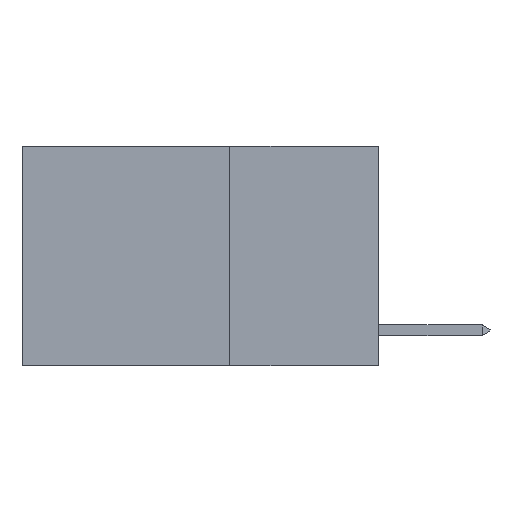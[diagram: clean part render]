
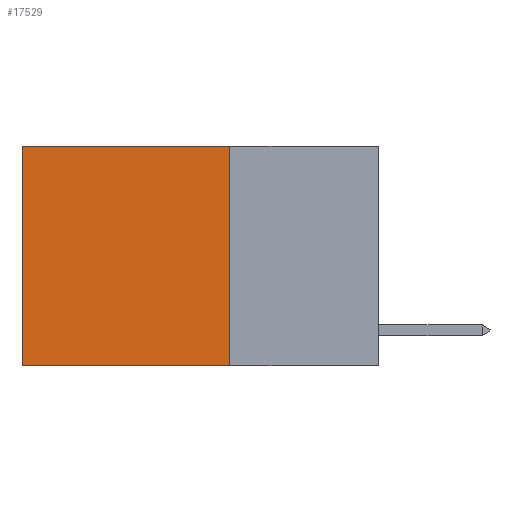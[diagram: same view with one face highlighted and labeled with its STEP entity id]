
A CAD part, left-side view. The second image highlights one B-rep face of the part: STEP entity #17529.
In plain terms, the highlighted planar face has unit normal (-1, 0, 0).
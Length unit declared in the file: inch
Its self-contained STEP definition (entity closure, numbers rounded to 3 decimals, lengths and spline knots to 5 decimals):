
#8 = CARTESIAN_POINT ( 'NONE',  ( 0.2625, 0.25, 0. ) ) ;
#123 = CARTESIAN_POINT ( 'NONE',  ( 0.2625, 0.6, 0. ) ) ;
#427 = VECTOR ( 'NONE', #13762, 39.37008 ) ;
#448 = DIRECTION ( 'NONE',  ( 1., 0., 0. ) ) ;
#703 = EDGE_CURVE ( 'NONE', #19741, #7677, #21095, .T. ) ;
#1011 = CARTESIAN_POINT ( 'NONE',  ( 0.2625, 0.25, 0. ) ) ;
#1373 = VECTOR ( 'NONE', #2758, 39.37008 ) ;
#1492 = CARTESIAN_POINT ( 'NONE',  ( 0.2625, 0.25, 0. ) ) ;
#1510 = ORIENTED_EDGE ( 'NONE', *, *, #703, .F. ) ;
#2489 = EDGE_CURVE ( 'NONE', #19741, #17463, #8851, .T. ) ;
#2511 = AXIS2_PLACEMENT_3D ( 'NONE', #8, #448, #7081 ) ;
#2758 = DIRECTION ( 'NONE',  ( 0., 0., -1. ) ) ;
#3025 = DIRECTION ( 'NONE',  ( 0., 0., -1. ) ) ;
#3809 = FACE_OUTER_BOUND ( 'NONE', #14700, .T. ) ;
#5686 = CARTESIAN_POINT ( 'NONE',  ( 0.2625, 0.6, -0.37 ) ) ;
#7005 = ORIENTED_EDGE ( 'NONE', *, *, #13951, .F. ) ;
#7081 = DIRECTION ( 'NONE',  ( 0., 0., -1. ) ) ;
#7677 = VERTEX_POINT ( 'NONE', #16591 ) ;
#7756 = LINE ( 'NONE', #15914, #13589 ) ;
#8752 = CARTESIAN_POINT ( 'NONE',  ( 0.2625, 0.25, 0. ) ) ;
#8851 = LINE ( 'NONE', #8752, #427 ) ;
#8890 = ORIENTED_EDGE ( 'NONE', *, *, #9875, .T. ) ;
#9255 = DIRECTION ( 'NONE',  ( 0., 1., 0. ) ) ;
#9875 = EDGE_CURVE ( 'NONE', #17463, #18696, #12842, .T. ) ;
#9918 = ORIENTED_EDGE ( 'NONE', *, *, #2489, .T. ) ;
#11668 = PLANE ( 'NONE',  #2511 ) ;
#12842 = LINE ( 'NONE', #17979, #17739 ) ;
#13589 = VECTOR ( 'NONE', #9255, 39.37008 ) ;
#13762 = DIRECTION ( 'NONE',  ( 0., 1., 0. ) ) ;
#13951 = EDGE_CURVE ( 'NONE', #7677, #18696, #7756, .T. ) ;
#14700 = EDGE_LOOP ( 'NONE', ( #8890, #7005, #1510, #9918 ) ) ;
#15914 = CARTESIAN_POINT ( 'NONE',  ( 0.2625, 0.25, -0.37 ) ) ;
#16591 = CARTESIAN_POINT ( 'NONE',  ( 0.2625, 0.25, -0.37 ) ) ;
#17463 = VERTEX_POINT ( 'NONE', #123 ) ;
#17529 = ADVANCED_FACE ( 'NONE', ( #3809 ), #11668, .F. ) ;
#17739 = VECTOR ( 'NONE', #3025, 39.37008 ) ;
#17979 = CARTESIAN_POINT ( 'NONE',  ( 0.2625, 0.6, 0. ) ) ;
#18696 = VERTEX_POINT ( 'NONE', #5686 ) ;
#19741 = VERTEX_POINT ( 'NONE', #1492 ) ;
#21095 = LINE ( 'NONE', #1011, #1373 ) ;
